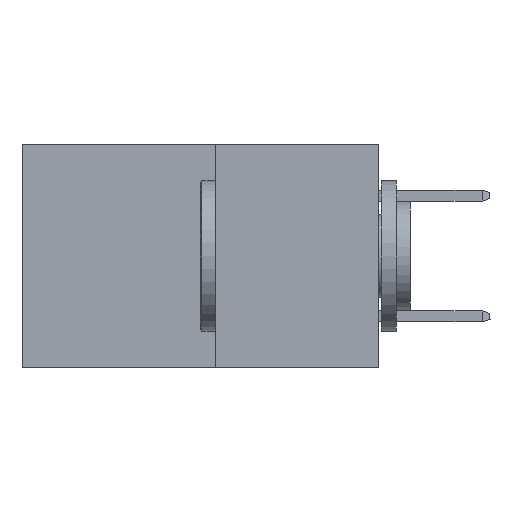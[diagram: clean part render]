
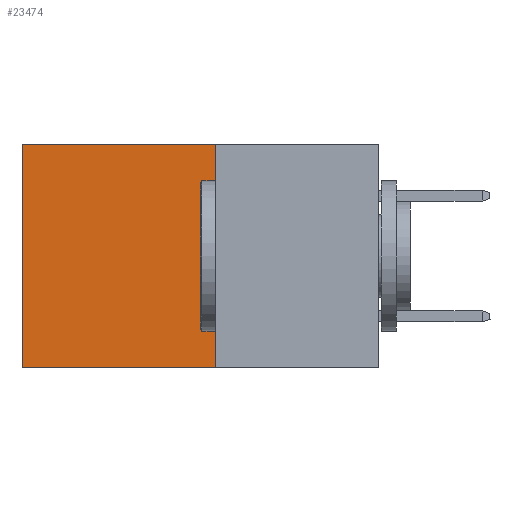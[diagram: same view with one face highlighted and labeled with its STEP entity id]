
A CAD part, left-side view. The second image highlights one B-rep face of the part: STEP entity #23474.
In plain terms, the highlighted planar face has unit normal (-1, 0, 0).
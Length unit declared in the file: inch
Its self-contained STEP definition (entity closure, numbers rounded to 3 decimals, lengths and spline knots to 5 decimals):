
#398 = ORIENTED_EDGE ( 'NONE', *, *, #13095, .T. ) ;
#1314 = LINE ( 'NONE', #20963, #11797 ) ;
#1751 = ORIENTED_EDGE ( 'NONE', *, *, #12143, .F. ) ;
#1905 = CARTESIAN_POINT ( 'NONE',  ( 0.277, 0.27, -0.37 ) ) ;
#2394 = CARTESIAN_POINT ( 'NONE',  ( 0.277, 0.59, -0.37 ) ) ;
#4076 = DIRECTION ( 'NONE',  ( 0., 0., -1. ) ) ;
#4237 = CARTESIAN_POINT ( 'NONE',  ( 0.277, 0.27, -0.37 ) ) ;
#5253 = VERTEX_POINT ( 'NONE', #14456 ) ;
#6308 = VECTOR ( 'NONE', #13423, 39.37008 ) ;
#6381 = ORIENTED_EDGE ( 'NONE', *, *, #12884, .T. ) ;
#6541 = EDGE_CURVE ( 'NONE', #11534, #5253, #23658, .T. ) ;
#6563 = DIRECTION ( 'NONE',  ( 1., 0., 0. ) ) ;
#6748 = CARTESIAN_POINT ( 'NONE',  ( 0.277, 0.27, -0.37 ) ) ;
#7516 = ORIENTED_EDGE ( 'NONE', *, *, #6541, .F. ) ;
#10147 = DIRECTION ( 'NONE',  ( 0., 1., 0. ) ) ;
#11534 = VERTEX_POINT ( 'NONE', #24675 ) ;
#11797 = VECTOR ( 'NONE', #10147, 39.37008 ) ;
#12143 = EDGE_CURVE ( 'NONE', #5253, #18384, #18297, .T. ) ;
#12150 = LINE ( 'NONE', #21982, #6308 ) ;
#12257 = VECTOR ( 'NONE', #4076, 39.37008 ) ;
#12538 = VECTOR ( 'NONE', #13364, 39.37008 ) ;
#12884 = EDGE_CURVE ( 'NONE', #25504, #18384, #12150, .T. ) ;
#13095 = EDGE_CURVE ( 'NONE', #11534, #25504, #1314, .T. ) ;
#13364 = DIRECTION ( 'NONE',  ( 0., 1., 0. ) ) ;
#13423 = DIRECTION ( 'NONE',  ( 0., 0., -1. ) ) ;
#14456 = CARTESIAN_POINT ( 'NONE',  ( 0.277, 0.27, -0.37 ) ) ;
#16213 = AXIS2_PLACEMENT_3D ( 'NONE', #1905, #6563, #21750 ) ;
#18297 = LINE ( 'NONE', #6748, #12538 ) ;
#18384 = VERTEX_POINT ( 'NONE', #2394 ) ;
#20963 = CARTESIAN_POINT ( 'NONE',  ( 0.277, 0.27, 0. ) ) ;
#21693 = CARTESIAN_POINT ( 'NONE',  ( 0.277, 0.59, 0. ) ) ;
#21750 = DIRECTION ( 'NONE',  ( 0., 0., -1. ) ) ;
#21921 = FACE_OUTER_BOUND ( 'NONE', #24747, .T. ) ;
#21982 = CARTESIAN_POINT ( 'NONE',  ( 0.277, 0.59, -0.37 ) ) ;
#23474 = ADVANCED_FACE ( 'NONE', ( #21921 ), #25852, .F. ) ;
#23658 = LINE ( 'NONE', #4237, #12257 ) ;
#24675 = CARTESIAN_POINT ( 'NONE',  ( 0.277, 0.27, 0. ) ) ;
#24747 = EDGE_LOOP ( 'NONE', ( #6381, #1751, #7516, #398 ) ) ;
#25504 = VERTEX_POINT ( 'NONE', #21693 ) ;
#25852 = PLANE ( 'NONE',  #16213 ) ;
